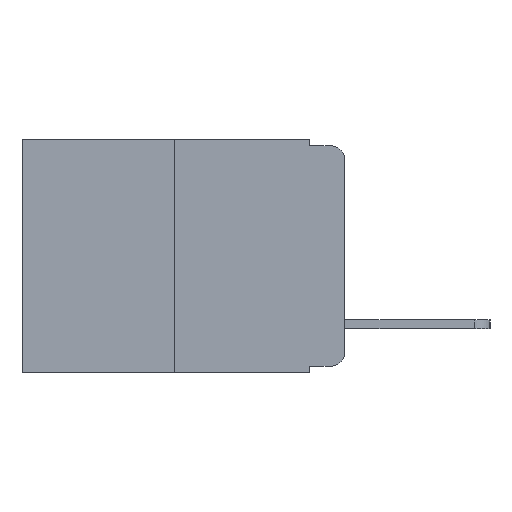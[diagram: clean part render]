
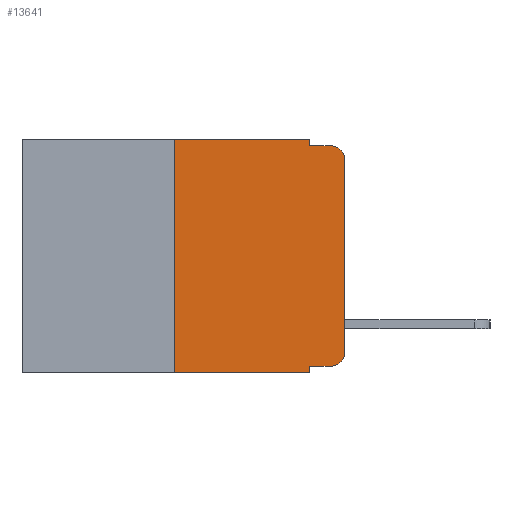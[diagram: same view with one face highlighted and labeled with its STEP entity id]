
A CAD part, left-side view. The second image highlights one B-rep face of the part: STEP entity #13641.
In plain terms, the highlighted planar face has unit normal (-1, 0, 0).
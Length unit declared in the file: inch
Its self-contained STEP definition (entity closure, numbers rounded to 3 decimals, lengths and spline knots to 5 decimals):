
#155 = CARTESIAN_POINT ( 'NONE',  ( 0., 0.02, -0.03 ) ) ;
#332 = CARTESIAN_POINT ( 'NONE',  ( 0., 0.051, 0. ) ) ;
#433 = ORIENTED_EDGE ( 'NONE', *, *, #11603, .T. ) ;
#638 = LINE ( 'NONE', #19270, #5053 ) ;
#646 = EDGE_CURVE ( 'NONE', #4731, #16708, #9083, .T. ) ;
#733 = DIRECTION ( 'NONE',  ( 0., -1., 0. ) ) ;
#813 = DIRECTION ( 'NONE',  ( 0., -1., 0. ) ) ;
#1809 = DIRECTION ( 'NONE',  ( 0., 0., 1. ) ) ;
#1828 = VERTEX_POINT ( 'NONE', #5000 ) ;
#1906 = DIRECTION ( 'NONE',  ( 0., 0., -1. ) ) ;
#2106 = EDGE_LOOP ( 'NONE', ( #15226, #12620, #12541, #6031, #9453, #6283, #7157, #15036, #2334, #433 ) ) ;
#2334 = ORIENTED_EDGE ( 'NONE', *, *, #20811, .T. ) ;
#2627 = VERTEX_POINT ( 'NONE', #3848 ) ;
#2685 = VECTOR ( 'NONE', #10011, 39.37008 ) ;
#2984 = CARTESIAN_POINT ( 'NONE',  ( 0., 0.051, -0.01 ) ) ;
#3510 = CARTESIAN_POINT ( 'NONE',  ( 0., 0.051, -0.333 ) ) ;
#3608 = DIRECTION ( 'NONE',  ( 0., 0., -1. ) ) ;
#3848 = CARTESIAN_POINT ( 'NONE',  ( 0., 0.051, -0.343 ) ) ;
#4321 = VECTOR ( 'NONE', #733, 39.37008 ) ;
#4731 = VERTEX_POINT ( 'NONE', #18018 ) ;
#5000 = CARTESIAN_POINT ( 'NONE',  ( 0., 0.02, -0.01 ) ) ;
#5053 = VECTOR ( 'NONE', #9753, 39.37008 ) ;
#5246 = FACE_OUTER_BOUND ( 'NONE', #2106, .T. ) ;
#5697 = EDGE_CURVE ( 'NONE', #11983, #4731, #6923, .T. ) ;
#5707 = CARTESIAN_POINT ( 'NONE',  ( 0., 0., -0.313 ) ) ;
#5708 = CARTESIAN_POINT ( 'NONE',  ( 0., 0.051, -0.333 ) ) ;
#6031 = ORIENTED_EDGE ( 'NONE', *, *, #10971, .F. ) ;
#6283 = ORIENTED_EDGE ( 'NONE', *, *, #5697, .F. ) ;
#6397 = CARTESIAN_POINT ( 'NONE',  ( 0., 0.02, -0.313 ) ) ;
#6923 = LINE ( 'NONE', #8380, #2685 ) ;
#7157 = ORIENTED_EDGE ( 'NONE', *, *, #11100, .T. ) ;
#7158 = DIRECTION ( 'NONE',  ( 1., 0., 0. ) ) ;
#7608 = VECTOR ( 'NONE', #1809, 39.37008 ) ;
#7777 = VECTOR ( 'NONE', #3608, 39.37008 ) ;
#7943 = CARTESIAN_POINT ( 'NONE',  ( 0., 0.02, -0.333 ) ) ;
#7978 = DIRECTION ( 'NONE',  ( 0., 0., -1. ) ) ;
#8059 = EDGE_CURVE ( 'NONE', #16362, #9961, #20316, .T. ) ;
#8334 = CIRCLE ( 'NONE', #16861, 0.02 ) ;
#8380 = CARTESIAN_POINT ( 'NONE',  ( 0., 0.25, 0. ) ) ;
#9083 = LINE ( 'NONE', #16734, #12392 ) ;
#9453 = ORIENTED_EDGE ( 'NONE', *, *, #646, .F. ) ;
#9753 = DIRECTION ( 'NONE',  ( 0., 0., -1. ) ) ;
#9842 = EDGE_CURVE ( 'NONE', #14094, #1828, #11340, .T. ) ;
#9961 = VERTEX_POINT ( 'NONE', #19215 ) ;
#10011 = DIRECTION ( 'NONE',  ( 0., 0., 1. ) ) ;
#10041 = CARTESIAN_POINT ( 'NONE',  ( 0., 0.051, 0. ) ) ;
#10345 = PLANE ( 'NONE',  #13742 ) ;
#10971 = EDGE_CURVE ( 'NONE', #16708, #14094, #16313, .T. ) ;
#11100 = EDGE_CURVE ( 'NONE', #11983, #2627, #12857, .T. ) ;
#11251 = EDGE_CURVE ( 'NONE', #12229, #2627, #638, .T. ) ;
#11340 = LINE ( 'NONE', #2984, #12352 ) ;
#11571 = DIRECTION ( 'NONE',  ( -1., 0., 0. ) ) ;
#11603 = EDGE_CURVE ( 'NONE', #19052, #16362, #16758, .T. ) ;
#11983 = VERTEX_POINT ( 'NONE', #16975 ) ;
#12100 = LINE ( 'NONE', #5708, #19503 ) ;
#12229 = VERTEX_POINT ( 'NONE', #3510 ) ;
#12352 = VECTOR ( 'NONE', #14182, 39.37008 ) ;
#12392 = VECTOR ( 'NONE', #20022, 39.37008 ) ;
#12541 = ORIENTED_EDGE ( 'NONE', *, *, #9842, .F. ) ;
#12620 = ORIENTED_EDGE ( 'NONE', *, *, #19939, .T. ) ;
#12857 = LINE ( 'NONE', #20014, #4321 ) ;
#13586 = CARTESIAN_POINT ( 'NONE',  ( 0., 0.473, 0. ) ) ;
#13641 = ADVANCED_FACE ( 'NONE', ( #5246 ), #10345, .F. ) ;
#13742 = AXIS2_PLACEMENT_3D ( 'NONE', #13586, #7158, #18346 ) ;
#14094 = VERTEX_POINT ( 'NONE', #17778 ) ;
#14182 = DIRECTION ( 'NONE',  ( 0., -1., 0. ) ) ;
#15036 = ORIENTED_EDGE ( 'NONE', *, *, #11251, .F. ) ;
#15226 = ORIENTED_EDGE ( 'NONE', *, *, #8059, .T. ) ;
#16313 = LINE ( 'NONE', #10041, #7777 ) ;
#16362 = VERTEX_POINT ( 'NONE', #5707 ) ;
#16708 = VERTEX_POINT ( 'NONE', #332 ) ;
#16734 = CARTESIAN_POINT ( 'NONE',  ( 0., 0.473, 0. ) ) ;
#16758 = CIRCLE ( 'NONE', #18202, 0.02 ) ;
#16861 = AXIS2_PLACEMENT_3D ( 'NONE', #155, #11571, #1906 ) ;
#16975 = CARTESIAN_POINT ( 'NONE',  ( 0., 0.25, -0.343 ) ) ;
#17570 = DIRECTION ( 'NONE',  ( -1., 0., 0. ) ) ;
#17778 = CARTESIAN_POINT ( 'NONE',  ( 0., 0.051, -0.01 ) ) ;
#18018 = CARTESIAN_POINT ( 'NONE',  ( 0., 0.25, 0. ) ) ;
#18202 = AXIS2_PLACEMENT_3D ( 'NONE', #6397, #17570, #7978 ) ;
#18346 = DIRECTION ( 'NONE',  ( 0., 0., -1. ) ) ;
#19052 = VERTEX_POINT ( 'NONE', #7943 ) ;
#19215 = CARTESIAN_POINT ( 'NONE',  ( 0., 0., -0.03 ) ) ;
#19270 = CARTESIAN_POINT ( 'NONE',  ( 0., 0.051, 0. ) ) ;
#19503 = VECTOR ( 'NONE', #813, 39.37008 ) ;
#19939 = EDGE_CURVE ( 'NONE', #9961, #1828, #8334, .T. ) ;
#20014 = CARTESIAN_POINT ( 'NONE',  ( 0., 0.473, -0.343 ) ) ;
#20022 = DIRECTION ( 'NONE',  ( 0., -1., 0. ) ) ;
#20316 = LINE ( 'NONE', #20848, #7608 ) ;
#20811 = EDGE_CURVE ( 'NONE', #12229, #19052, #12100, .T. ) ;
#20848 = CARTESIAN_POINT ( 'NONE',  ( 0., 0., 0. ) ) ;
